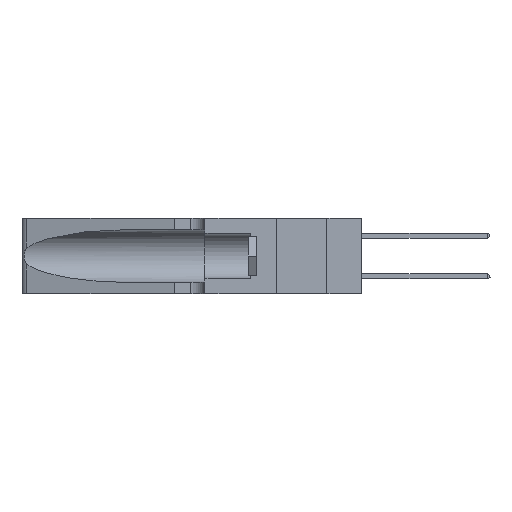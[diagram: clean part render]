
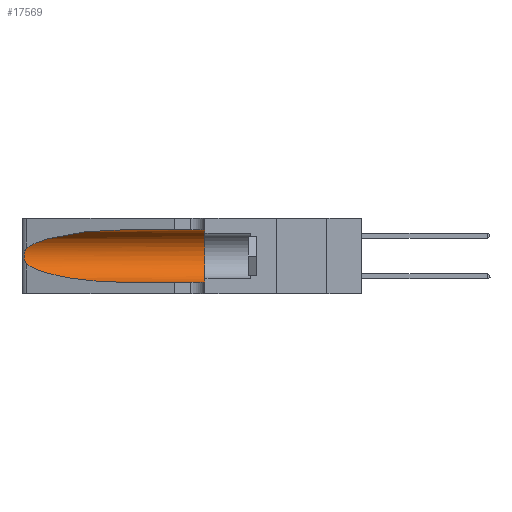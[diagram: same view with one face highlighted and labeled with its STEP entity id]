
A CAD part, left-side view. The second image highlights one B-rep face of the part: STEP entity #17569.
In plain terms, the highlighted cylindrical face has radius 3.308 mm (diameter 6.617 mm), a partial arc.
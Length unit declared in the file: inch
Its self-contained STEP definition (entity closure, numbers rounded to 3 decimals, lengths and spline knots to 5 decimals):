
#562 = ORIENTED_EDGE ( 'NONE', *, *, #1684, .T. ) ;
#1684 = EDGE_CURVE ( 'NONE', #4235, #25309, #9524, .T. ) ;
#2855 = EDGE_CURVE ( 'NONE', #4235, #4179, #10989, .T. ) ;
#4079 = CARTESIAN_POINT ( 'NONE',  ( 0.18966, 0.96281, 0.31525 ) ) ;
#4178 = EDGE_LOOP ( 'NONE', ( #562, #20250, #20396, #27210, #29527, #6715 ) ) ;
#4179 = VERTEX_POINT ( 'NONE', #24160 ) ;
#4235 = VERTEX_POINT ( 'NONE', #8279 ) ;
#4710 = AXIS2_PLACEMENT_3D ( 'NONE', #22577, #8070, #22683 ) ;
#5553 = FACE_OUTER_BOUND ( 'NONE', #4178, .T. ) ;
#6623 = CARTESIAN_POINT ( 'NONE',  ( 0.26017, 1.23833, 0.17102 ) ) ;
#6715 = ORIENTED_EDGE ( 'NONE', *, *, #2855, .F. ) ;
#6974 = DIRECTION ( 'NONE',  ( 0., -1., 0. ) ) ;
#7654 = AXIS2_PLACEMENT_3D ( 'NONE', #20105, #8037, #22647 ) ;
#8037 = DIRECTION ( 'NONE',  ( 0., 1., 0. ) ) ;
#8042 = CARTESIAN_POINT ( 'NONE',  ( 0.18966, 0.96281, 0.05475 ) ) ;
#8070 = DIRECTION ( 'NONE',  ( 0., -1., 0. ) ) ;
#8279 = CARTESIAN_POINT ( 'NONE',  ( 0.1305, 0.72297, 0.31525 ) ) ;
#9524 =( BOUNDED_CURVE ( )  B_SPLINE_CURVE ( 3, ( #25836, #4079, #16252, #28997 ),
 .UNSPECIFIED., .F., .T. ) 
 B_SPLINE_CURVE_WITH_KNOTS ( ( 4, 4 ),
 ( 1.5708, 2.84003 ),
 .UNSPECIFIED. ) 
 CURVE ( )  GEOMETRIC_REPRESENTATION_ITEM ( )  RATIONAL_B_SPLINE_CURVE ( ( 1., 0.87, 0.87, 1. ) ) 
 REPRESENTATION_ITEM ( '' )  );
#9892 = B_SPLINE_CURVE_WITH_KNOTS ( 'NONE', 3,
 ( #11391, #23914, #21109, #14232, #23687, #11806, #14135, #11598, #6623, #16348, #21322, #20996, #28557, #14020 ),
 .UNSPECIFIED., .F., .F.,
 ( 4, 2, 2, 2, 2, 2, 4 ),
 ( 0., 0.00027, 0.00053, 0.00107, 0.0016, 0.00187, 0.00214 ),
 .UNSPECIFIED. ) ;
#10343 = VECTOR ( 'NONE', #11510, 39.37008 ) ;
#10584 = CARTESIAN_POINT ( 'NONE',  ( 0.2373, 1.15595, 0.08982 ) ) ;
#10989 = LINE ( 'NONE', #23843, #20838 ) ;
#11110 = CIRCLE ( 'NONE', #7654, 0.13025 ) ;
#11391 = CARTESIAN_POINT ( 'NONE',  ( 0.25487, 1.22718, 0.22369 ) ) ;
#11510 = DIRECTION ( 'NONE',  ( 0., -1., 0. ) ) ;
#11598 = CARTESIAN_POINT ( 'NONE',  ( 0.26075, 1.23896, 0.178 ) ) ;
#11806 = CARTESIAN_POINT ( 'NONE',  ( 0.26018, 1.23835, 0.19895 ) ) ;
#12927 = CARTESIAN_POINT ( 'NONE',  ( 0.1305, 0.72297, 0.05475 ) ) ;
#12992 = EDGE_CURVE ( 'NONE', #4179, #14381, #11110, .T. ) ;
#14020 = CARTESIAN_POINT ( 'NONE',  ( 0.25487, 1.22718, 0.14631 ) ) ;
#14135 = CARTESIAN_POINT ( 'NONE',  ( 0.26075, 1.23896, 0.19203 ) ) ;
#14232 = CARTESIAN_POINT ( 'NONE',  ( 0.25787, 1.23484, 0.2124 ) ) ;
#14381 = VERTEX_POINT ( 'NONE', #17975 ) ;
#15150 = CARTESIAN_POINT ( 'NONE',  ( 0.1305, 0.72297, 0.05475 ) ) ;
#15262 = VERTEX_POINT ( 'NONE', #15150 ) ;
#15602 = VERTEX_POINT ( 'NONE', #23872 ) ;
#16252 = CARTESIAN_POINT ( 'NONE',  ( 0.2373, 1.15595, 0.28018 ) ) ;
#16348 = CARTESIAN_POINT ( 'NONE',  ( 0.25856, 1.23593, 0.16098 ) ) ;
#17569 = ADVANCED_FACE ( 'NONE', ( #5553 ), #29815, .F. ) ;
#17975 = CARTESIAN_POINT ( 'NONE',  ( 0.1305, 0.35, 0.05475 ) ) ;
#19765 = CARTESIAN_POINT ( 'NONE',  ( 0.25487, 1.22718, 0.22369 ) ) ;
#20105 = CARTESIAN_POINT ( 'NONE',  ( 0.1305, 0.35, 0.185 ) ) ;
#20250 = ORIENTED_EDGE ( 'NONE', *, *, #30407, .T. ) ;
#20396 = ORIENTED_EDGE ( 'NONE', *, *, #30776, .T. ) ;
#20838 = VECTOR ( 'NONE', #6974, 39.37008 ) ;
#20996 = CARTESIAN_POINT ( 'NONE',  ( 0.25639, 1.23186, 0.15144 ) ) ;
#21109 = CARTESIAN_POINT ( 'NONE',  ( 0.25639, 1.23184, 0.21858 ) ) ;
#21322 = CARTESIAN_POINT ( 'NONE',  ( 0.25789, 1.23486, 0.15765 ) ) ;
#22577 = CARTESIAN_POINT ( 'NONE',  ( 0.1305, 1.61858, 0.185 ) ) ;
#22647 = DIRECTION ( 'NONE',  ( 0., 0., 1. ) ) ;
#22683 = DIRECTION ( 'NONE',  ( 0., 0., -1. ) ) ;
#22869 = EDGE_CURVE ( 'NONE', #15262, #14381, #24068, .T. ) ;
#23524 =( BOUNDED_CURVE ( )  B_SPLINE_CURVE ( 3, ( #25116, #10584, #8042, #12927 ),
 .UNSPECIFIED., .F., .T. ) 
 B_SPLINE_CURVE_WITH_KNOTS ( ( 4, 4 ),
 ( 3.44316, 4.71239 ),
 .UNSPECIFIED. ) 
 CURVE ( )  GEOMETRIC_REPRESENTATION_ITEM ( )  RATIONAL_B_SPLINE_CURVE ( ( 1., 0.87, 0.87, 1. ) ) 
 REPRESENTATION_ITEM ( '' )  );
#23687 = CARTESIAN_POINT ( 'NONE',  ( 0.25854, 1.2359, 0.20912 ) ) ;
#23843 = CARTESIAN_POINT ( 'NONE',  ( 0.1305, 1.61858, 0.31525 ) ) ;
#23872 = CARTESIAN_POINT ( 'NONE',  ( 0.25487, 1.22718, 0.14631 ) ) ;
#23914 = CARTESIAN_POINT ( 'NONE',  ( 0.25555, 1.22994, 0.2215 ) ) ;
#24068 = LINE ( 'NONE', #29054, #10343 ) ;
#24160 = CARTESIAN_POINT ( 'NONE',  ( 0.1305, 0.35, 0.31525 ) ) ;
#25116 = CARTESIAN_POINT ( 'NONE',  ( 0.25487, 1.22718, 0.14631 ) ) ;
#25309 = VERTEX_POINT ( 'NONE', #19765 ) ;
#25836 = CARTESIAN_POINT ( 'NONE',  ( 0.1305, 0.72297, 0.31525 ) ) ;
#27210 = ORIENTED_EDGE ( 'NONE', *, *, #22869, .T. ) ;
#28557 = CARTESIAN_POINT ( 'NONE',  ( 0.25555, 1.22993, 0.14849 ) ) ;
#28997 = CARTESIAN_POINT ( 'NONE',  ( 0.25487, 1.22718, 0.22369 ) ) ;
#29054 = CARTESIAN_POINT ( 'NONE',  ( 0.1305, 1.61858, 0.05475 ) ) ;
#29527 = ORIENTED_EDGE ( 'NONE', *, *, #12992, .F. ) ;
#29815 = CYLINDRICAL_SURFACE ( 'NONE', #4710, 0.13025 ) ;
#30407 = EDGE_CURVE ( 'NONE', #25309, #15602, #9892, .T. ) ;
#30776 = EDGE_CURVE ( 'NONE', #15602, #15262, #23524, .T. ) ;
